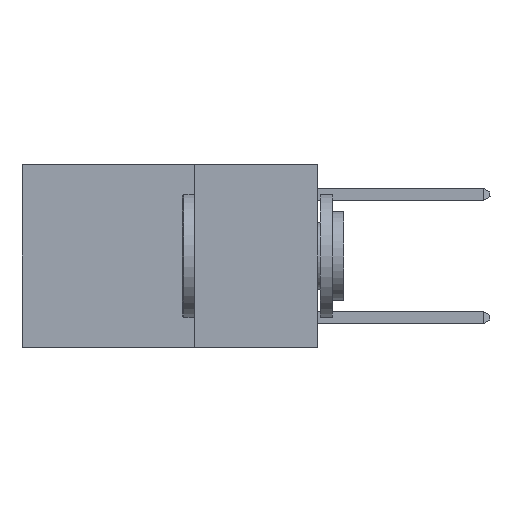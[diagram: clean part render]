
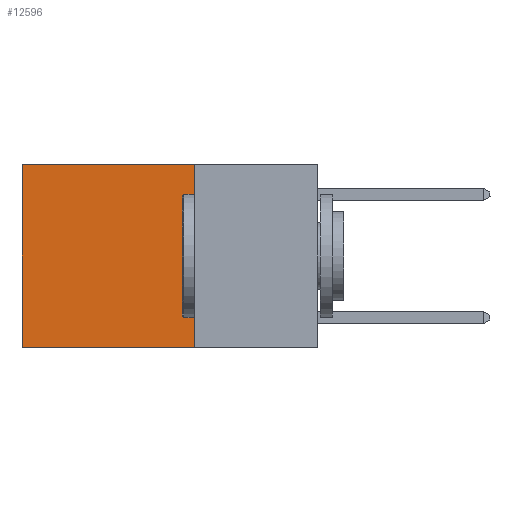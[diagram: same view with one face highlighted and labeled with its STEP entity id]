
A CAD part, left-side view. The second image highlights one B-rep face of the part: STEP entity #12596.
In plain terms, the highlighted planar face has unit normal (-1, 0, 0).
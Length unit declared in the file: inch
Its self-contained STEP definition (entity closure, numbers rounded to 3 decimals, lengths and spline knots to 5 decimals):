
#117 = ORIENTED_EDGE ( 'NONE', *, *, #19600, .T. ) ;
#788 = LINE ( 'NONE', #20228, #24070 ) ;
#1786 = VECTOR ( 'NONE', #5344, 39.37008 ) ;
#2254 = CARTESIAN_POINT ( 'NONE',  ( 0.2625, 0.25, 0. ) ) ;
#2725 = VERTEX_POINT ( 'NONE', #15296 ) ;
#3933 = CARTESIAN_POINT ( 'NONE',  ( 0.2625, 0.6, -0.37 ) ) ;
#4478 = DIRECTION ( 'NONE',  ( 0., 1., 0. ) ) ;
#5263 = CARTESIAN_POINT ( 'NONE',  ( 0.2625, 0.25, 0. ) ) ;
#5344 = DIRECTION ( 'NONE',  ( 0., 0., -1. ) ) ;
#6602 = CARTESIAN_POINT ( 'NONE',  ( 0.2625, 0.6, 0. ) ) ;
#7293 = AXIS2_PLACEMENT_3D ( 'NONE', #19071, #24094, #18384 ) ;
#7603 = EDGE_CURVE ( 'NONE', #22721, #2725, #25003, .T. ) ;
#7743 = CARTESIAN_POINT ( 'NONE',  ( 0.2625, 0.25, 0. ) ) ;
#7924 = ORIENTED_EDGE ( 'NONE', *, *, #21200, .F. ) ;
#8454 = EDGE_LOOP ( 'NONE', ( #117, #18660, #7924, #17133 ) ) ;
#10266 = FACE_OUTER_BOUND ( 'NONE', #8454, .T. ) ;
#11751 = DIRECTION ( 'NONE',  ( 0., 0., -1. ) ) ;
#12020 = CARTESIAN_POINT ( 'NONE',  ( 0.2625, 0.25, -0.37 ) ) ;
#12596 = ADVANCED_FACE ( 'NONE', ( #10266 ), #19751, .F. ) ;
#13627 = VERTEX_POINT ( 'NONE', #12020 ) ;
#14976 = VECTOR ( 'NONE', #21354, 39.37008 ) ;
#15296 = CARTESIAN_POINT ( 'NONE',  ( 0.2625, 0.6, 0. ) ) ;
#15376 = VERTEX_POINT ( 'NONE', #3933 ) ;
#15881 = VECTOR ( 'NONE', #11751, 39.37008 ) ;
#17133 = ORIENTED_EDGE ( 'NONE', *, *, #7603, .T. ) ;
#18384 = DIRECTION ( 'NONE',  ( 0., 0., -1. ) ) ;
#18660 = ORIENTED_EDGE ( 'NONE', *, *, #24258, .F. ) ;
#18687 = LINE ( 'NONE', #7743, #15881 ) ;
#19071 = CARTESIAN_POINT ( 'NONE',  ( 0.2625, 0.25, 0. ) ) ;
#19600 = EDGE_CURVE ( 'NONE', #2725, #15376, #26022, .T. ) ;
#19751 = PLANE ( 'NONE',  #7293 ) ;
#20228 = CARTESIAN_POINT ( 'NONE',  ( 0.2625, 0.25, -0.37 ) ) ;
#21200 = EDGE_CURVE ( 'NONE', #22721, #13627, #18687, .T. ) ;
#21354 = DIRECTION ( 'NONE',  ( 0., 1., 0. ) ) ;
#22721 = VERTEX_POINT ( 'NONE', #2254 ) ;
#24070 = VECTOR ( 'NONE', #4478, 39.37008 ) ;
#24094 = DIRECTION ( 'NONE',  ( 1., 0., 0. ) ) ;
#24258 = EDGE_CURVE ( 'NONE', #13627, #15376, #788, .T. ) ;
#25003 = LINE ( 'NONE', #5263, #14976 ) ;
#26022 = LINE ( 'NONE', #6602, #1786 ) ;
